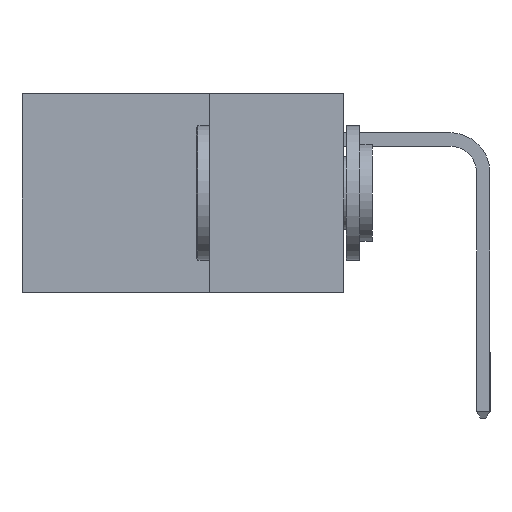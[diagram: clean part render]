
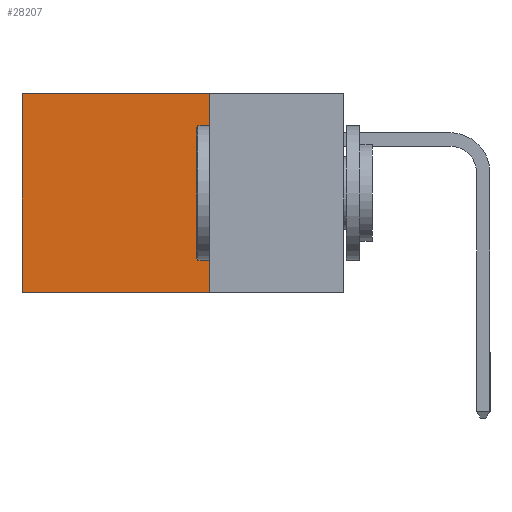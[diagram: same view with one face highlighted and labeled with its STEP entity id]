
A CAD part, left-side view. The second image highlights one B-rep face of the part: STEP entity #28207.
In plain terms, the highlighted planar face has unit normal (-1, 0, 0).
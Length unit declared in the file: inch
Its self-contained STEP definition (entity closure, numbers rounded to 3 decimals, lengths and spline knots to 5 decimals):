
#1988 = DIRECTION ( 'NONE',  ( 0., 1., 0. ) ) ;
#2190 = LINE ( 'NONE', #30747, #26872 ) ;
#4162 = PLANE ( 'NONE',  #28359 ) ;
#6294 = DIRECTION ( 'NONE',  ( 0., 1., 0. ) ) ;
#7758 = EDGE_CURVE ( 'NONE', #17348, #10828, #13808, .T. ) ;
#8640 = ORIENTED_EDGE ( 'NONE', *, *, #7758, .F. ) ;
#9177 = CARTESIAN_POINT ( 'NONE',  ( 0.298, 0.25, 0. ) ) ;
#10554 = ORIENTED_EDGE ( 'NONE', *, *, #23054, .T. ) ;
#10828 = VERTEX_POINT ( 'NONE', #26602 ) ;
#11120 = VERTEX_POINT ( 'NONE', #24238 ) ;
#11650 = DIRECTION ( 'NONE',  ( 0., 0., -1. ) ) ;
#12538 = DIRECTION ( 'NONE',  ( 0., 0., -1. ) ) ;
#12856 = CARTESIAN_POINT ( 'NONE',  ( 0.298, 0.25, 0. ) ) ;
#12871 = VECTOR ( 'NONE', #1988, 39.37008 ) ;
#13808 = LINE ( 'NONE', #12856, #31776 ) ;
#14679 = EDGE_LOOP ( 'NONE', ( #20788, #31703, #8640, #10554 ) ) ;
#15259 = VECTOR ( 'NONE', #19645, 39.37008 ) ;
#16823 = CARTESIAN_POINT ( 'NONE',  ( 0.298, 0.25, 0. ) ) ;
#17348 = VERTEX_POINT ( 'NONE', #18513 ) ;
#18513 = CARTESIAN_POINT ( 'NONE',  ( 0.298, 0.25, 0. ) ) ;
#19645 = DIRECTION ( 'NONE',  ( 0., 0., -1. ) ) ;
#20788 = ORIENTED_EDGE ( 'NONE', *, *, #23826, .T. ) ;
#21732 = LINE ( 'NONE', #29422, #15259 ) ;
#23054 = EDGE_CURVE ( 'NONE', #17348, #29676, #31604, .T. ) ;
#23826 = EDGE_CURVE ( 'NONE', #29676, #11120, #21732, .T. ) ;
#24238 = CARTESIAN_POINT ( 'NONE',  ( 0.298, 0.6, -0.37 ) ) ;
#26294 = DIRECTION ( 'NONE',  ( 1., 0., 0. ) ) ;
#26602 = CARTESIAN_POINT ( 'NONE',  ( 0.298, 0.25, -0.37 ) ) ;
#26686 = CARTESIAN_POINT ( 'NONE',  ( 0.298, 0.6, 0. ) ) ;
#26872 = VECTOR ( 'NONE', #6294, 39.37008 ) ;
#27445 = FACE_OUTER_BOUND ( 'NONE', #14679, .T. ) ;
#28207 = ADVANCED_FACE ( 'NONE', ( #27445 ), #4162, .F. ) ;
#28359 = AXIS2_PLACEMENT_3D ( 'NONE', #9177, #26294, #11650 ) ;
#29422 = CARTESIAN_POINT ( 'NONE',  ( 0.298, 0.6, 0. ) ) ;
#29676 = VERTEX_POINT ( 'NONE', #26686 ) ;
#30747 = CARTESIAN_POINT ( 'NONE',  ( 0.298, 0.25, -0.37 ) ) ;
#31357 = EDGE_CURVE ( 'NONE', #10828, #11120, #2190, .T. ) ;
#31604 = LINE ( 'NONE', #16823, #12871 ) ;
#31703 = ORIENTED_EDGE ( 'NONE', *, *, #31357, .F. ) ;
#31776 = VECTOR ( 'NONE', #12538, 39.37008 ) ;
